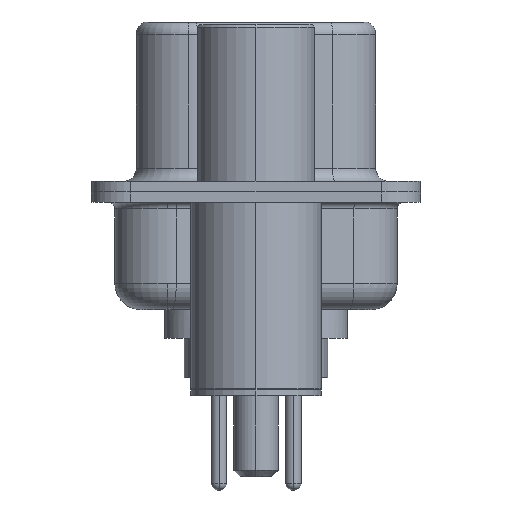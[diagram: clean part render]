
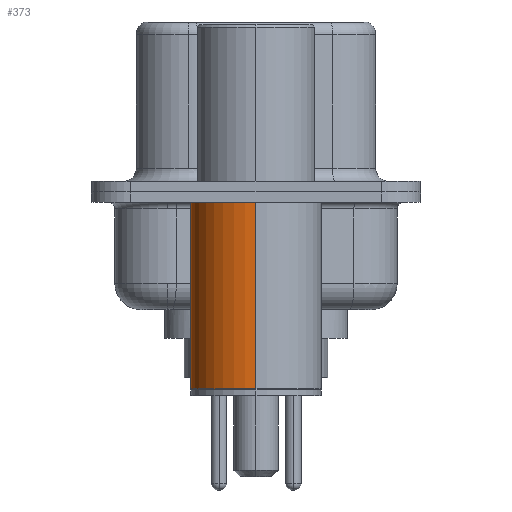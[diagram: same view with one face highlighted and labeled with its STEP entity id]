
A CAD part, left-side view. The second image highlights one B-rep face of the part: STEP entity #373.
In plain terms, the highlighted cylindrical face has radius 2.5 mm (diameter 5 mm), a partial arc.
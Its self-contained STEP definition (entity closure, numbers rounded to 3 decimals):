
#373 = ADVANCED_FACE ( 'NONE', ( #5683 ), #8886, .T. ) ;
#778 = CARTESIAN_POINT ( 'NONE',  ( -2.5, 0., 0.581 ) ) ;
#1480 = ORIENTED_EDGE ( 'NONE', *, *, #14443, .F. ) ;
#1968 = LINE ( 'NONE', #5244, #14961 ) ;
#3494 = CARTESIAN_POINT ( 'NONE',  ( 0., 0., 0.581 ) ) ;
#3530 = CIRCLE ( 'NONE', #17030, 2.5 ) ;
#3571 = CARTESIAN_POINT ( 'NONE',  ( 0., 0., -0.4 ) ) ;
#3992 = CARTESIAN_POINT ( 'NONE',  ( -2.5, 0., -7.525 ) ) ;
#4269 = DIRECTION ( 'NONE',  ( 0., 0., 1. ) ) ;
#4354 = CARTESIAN_POINT ( 'NONE',  ( 2.5, 0., -7.525 ) ) ;
#4976 = DIRECTION ( 'NONE',  ( 1., 0., 0. ) ) ;
#5244 = CARTESIAN_POINT ( 'NONE',  ( 2.5, 0., 0.581 ) ) ;
#5683 = FACE_OUTER_BOUND ( 'NONE', #6384, .T. ) ;
#5745 = CARTESIAN_POINT ( 'NONE',  ( -2.5, 0., -0.4 ) ) ;
#6384 = EDGE_LOOP ( 'NONE', ( #13233, #17440, #1480, #14406 ) ) ;
#7587 = AXIS2_PLACEMENT_3D ( 'NONE', #3494, #8008, #9034 ) ;
#7763 = DIRECTION ( 'NONE',  ( 0., 0., 1. ) ) ;
#8008 = DIRECTION ( 'NONE',  ( 0., 0., 1. ) ) ;
#8103 = AXIS2_PLACEMENT_3D ( 'NONE', #3571, #12913, #4976 ) ;
#8886 = CYLINDRICAL_SURFACE ( 'NONE', #7587, 2.5 ) ;
#9034 = DIRECTION ( 'NONE',  ( 1., 0., 0. ) ) ;
#9713 = VECTOR ( 'NONE', #7763, 1000. ) ;
#9886 = CARTESIAN_POINT ( 'NONE',  ( 2.5, 0., -0.4 ) ) ;
#10818 = EDGE_CURVE ( 'NONE', #16486, #16308, #3530, .T. ) ;
#11354 = EDGE_CURVE ( 'NONE', #16308, #16500, #16625, .T. ) ;
#11571 = EDGE_CURVE ( 'NONE', #16486, #14146, #1968, .T. ) ;
#12260 = CARTESIAN_POINT ( 'NONE',  ( 0., 0., -7.525 ) ) ;
#12913 = DIRECTION ( 'NONE',  ( 0., 0., 1. ) ) ;
#13233 = ORIENTED_EDGE ( 'NONE', *, *, #10818, .T. ) ;
#13567 = DIRECTION ( 'NONE',  ( 1., 0., 0. ) ) ;
#14146 = VERTEX_POINT ( 'NONE', #9886 ) ;
#14283 = CIRCLE ( 'NONE', #8103, 2.5 ) ;
#14406 = ORIENTED_EDGE ( 'NONE', *, *, #11571, .F. ) ;
#14443 = EDGE_CURVE ( 'NONE', #14146, #16500, #14283, .T. ) ;
#14961 = VECTOR ( 'NONE', #15831, 1000. ) ;
#15831 = DIRECTION ( 'NONE',  ( 0., 0., 1. ) ) ;
#16308 = VERTEX_POINT ( 'NONE', #3992 ) ;
#16486 = VERTEX_POINT ( 'NONE', #4354 ) ;
#16500 = VERTEX_POINT ( 'NONE', #5745 ) ;
#16625 = LINE ( 'NONE', #778, #9713 ) ;
#17030 = AXIS2_PLACEMENT_3D ( 'NONE', #12260, #4269, #13567 ) ;
#17440 = ORIENTED_EDGE ( 'NONE', *, *, #11354, .T. ) ;
